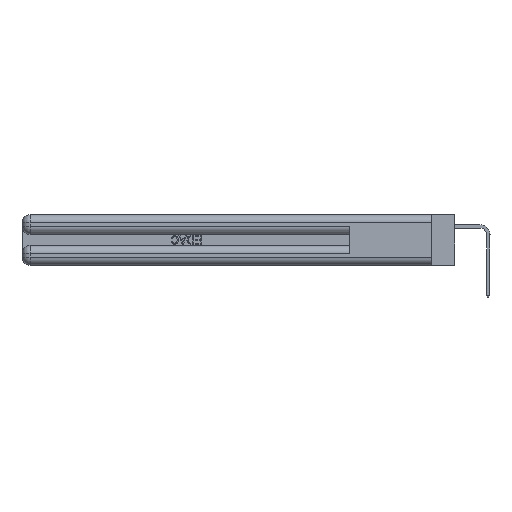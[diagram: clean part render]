
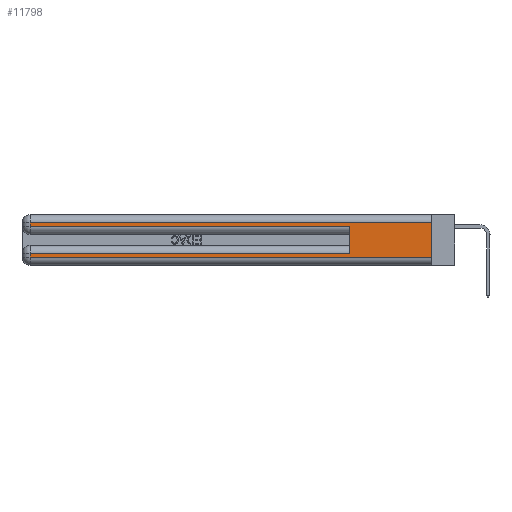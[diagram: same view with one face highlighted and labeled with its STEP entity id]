
A CAD part, left-side view. The second image highlights one B-rep face of the part: STEP entity #11798.
In plain terms, the highlighted planar face has unit normal (-1, 0, 0).
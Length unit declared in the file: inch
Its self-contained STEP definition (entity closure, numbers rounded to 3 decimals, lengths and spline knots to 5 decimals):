
#372 = VERTEX_POINT ( 'NONE', #23895 ) ;
#876 = EDGE_CURVE ( 'NONE', #7677, #9743, #2712, .T. ) ;
#1014 = EDGE_CURVE ( 'NONE', #28076, #23178, #6692, .T. ) ;
#1249 = VERTEX_POINT ( 'NONE', #17745 ) ;
#1571 = VECTOR ( 'NONE', #29913, 39.37008 ) ;
#2712 = LINE ( 'NONE', #8599, #1571 ) ;
#3788 = CARTESIAN_POINT ( 'NONE',  ( 0., 0., 0.37 ) ) ;
#5442 = ORIENTED_EDGE ( 'NONE', *, *, #15242, .T. ) ;
#6692 = LINE ( 'NONE', #34142, #24553 ) ;
#7235 = CARTESIAN_POINT ( 'NONE',  ( 0., 0.6, 0.145 ) ) ;
#7677 = VERTEX_POINT ( 'NONE', #22195 ) ;
#8266 = CARTESIAN_POINT ( 'NONE',  ( 0., 2.94, 0.37 ) ) ;
#8423 = LINE ( 'NONE', #7235, #26222 ) ;
#8599 = CARTESIAN_POINT ( 'NONE',  ( 0., 0., 0.285 ) ) ;
#9743 = VERTEX_POINT ( 'NONE', #9805 ) ;
#9805 = CARTESIAN_POINT ( 'NONE',  ( 0., 0.6, 0.285 ) ) ;
#10433 = CARTESIAN_POINT ( 'NONE',  ( 0., 0., 0.06 ) ) ;
#10852 = DIRECTION ( 'NONE',  ( 0., 0., 1. ) ) ;
#11050 = PLANE ( 'NONE',  #21343 ) ;
#11798 = ADVANCED_FACE ( 'NONE', ( #30178 ), #11050, .F. ) ;
#12207 = LINE ( 'NONE', #28104, #32257 ) ;
#12406 = LINE ( 'NONE', #39997, #39712 ) ;
#13673 = VERTEX_POINT ( 'NONE', #39233 ) ;
#14041 = ORIENTED_EDGE ( 'NONE', *, *, #26485, .T. ) ;
#14294 = ORIENTED_EDGE ( 'NONE', *, *, #25500, .T. ) ;
#14632 = DIRECTION ( 'NONE',  ( 0., 0., -1. ) ) ;
#14890 = VECTOR ( 'NONE', #36231, 39.37008 ) ;
#15242 = EDGE_CURVE ( 'NONE', #372, #1249, #43295, .T. ) ;
#16392 = DIRECTION ( 'NONE',  ( 0., 1., 0. ) ) ;
#17745 = CARTESIAN_POINT ( 'NONE',  ( 0., 2.94, 0.06 ) ) ;
#18469 = CARTESIAN_POINT ( 'NONE',  ( 0., 2.94, 0.37 ) ) ;
#19263 = CARTESIAN_POINT ( 'NONE',  ( 0., 0., 0.31 ) ) ;
#19550 = LINE ( 'NONE', #37977, #28996 ) ;
#20199 = DIRECTION ( 'NONE',  ( 0., -1., 0. ) ) ;
#21343 = AXIS2_PLACEMENT_3D ( 'NONE', #3788, #35951, #14632 ) ;
#22195 = CARTESIAN_POINT ( 'NONE',  ( 0., 2.94, 0.285 ) ) ;
#23178 = VERTEX_POINT ( 'NONE', #36043 ) ;
#23895 = CARTESIAN_POINT ( 'NONE',  ( 0., 2.94, 0.085 ) ) ;
#24553 = VECTOR ( 'NONE', #16392, 39.37008 ) ;
#25500 = EDGE_CURVE ( 'NONE', #13673, #372, #12406, .T. ) ;
#26222 = VECTOR ( 'NONE', #10852, 39.37008 ) ;
#26485 = EDGE_CURVE ( 'NONE', #1249, #32841, #19550, .T. ) ;
#28076 = VERTEX_POINT ( 'NONE', #19263 ) ;
#28104 = CARTESIAN_POINT ( 'NONE',  ( 0., 0., 0.37 ) ) ;
#28996 = VECTOR ( 'NONE', #20199, 39.37008 ) ;
#29576 = DIRECTION ( 'NONE',  ( 0., 0., -1. ) ) ;
#29913 = DIRECTION ( 'NONE',  ( 0., -1., 0. ) ) ;
#30178 = FACE_OUTER_BOUND ( 'NONE', #31911, .T. ) ;
#30243 = ORIENTED_EDGE ( 'NONE', *, *, #38408, .F. ) ;
#30929 = VECTOR ( 'NONE', #29576, 39.37008 ) ;
#31317 = EDGE_CURVE ( 'NONE', #23178, #7677, #40446, .T. ) ;
#31911 = EDGE_LOOP ( 'NONE', ( #30243, #35801, #44159, #44233, #33384, #14294, #5442, #14041 ) ) ;
#32257 = VECTOR ( 'NONE', #38922, 39.37008 ) ;
#32841 = VERTEX_POINT ( 'NONE', #10433 ) ;
#33384 = ORIENTED_EDGE ( 'NONE', *, *, #33579, .F. ) ;
#33579 = EDGE_CURVE ( 'NONE', #13673, #9743, #8423, .T. ) ;
#34142 = CARTESIAN_POINT ( 'NONE',  ( 0., 0., 0.31 ) ) ;
#35801 = ORIENTED_EDGE ( 'NONE', *, *, #1014, .T. ) ;
#35951 = DIRECTION ( 'NONE',  ( 1., 0., 0. ) ) ;
#36043 = CARTESIAN_POINT ( 'NONE',  ( 0., 2.94, 0.31 ) ) ;
#36231 = DIRECTION ( 'NONE',  ( 0., 0., -1. ) ) ;
#37977 = CARTESIAN_POINT ( 'NONE',  ( 0., 0., 0.06 ) ) ;
#38408 = EDGE_CURVE ( 'NONE', #28076, #32841, #12207, .T. ) ;
#38922 = DIRECTION ( 'NONE',  ( 0., 0., -1. ) ) ;
#39233 = CARTESIAN_POINT ( 'NONE',  ( 0., 0.6, 0.085 ) ) ;
#39712 = VECTOR ( 'NONE', #43564, 39.37008 ) ;
#39997 = CARTESIAN_POINT ( 'NONE',  ( 0., 0., 0.085 ) ) ;
#40446 = LINE ( 'NONE', #8266, #30929 ) ;
#43295 = LINE ( 'NONE', #18469, #14890 ) ;
#43564 = DIRECTION ( 'NONE',  ( 0., 1., 0. ) ) ;
#44159 = ORIENTED_EDGE ( 'NONE', *, *, #31317, .T. ) ;
#44233 = ORIENTED_EDGE ( 'NONE', *, *, #876, .T. ) ;
